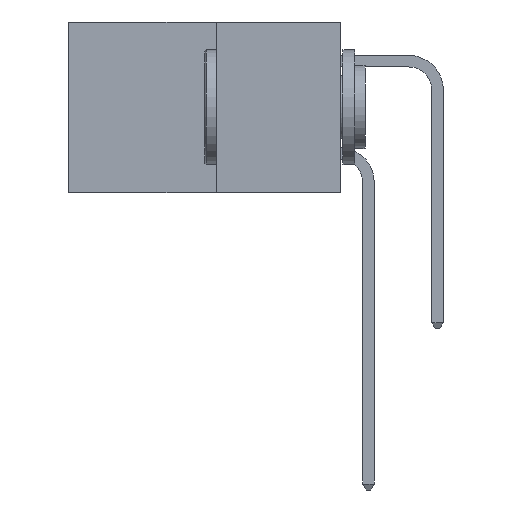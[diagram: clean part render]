
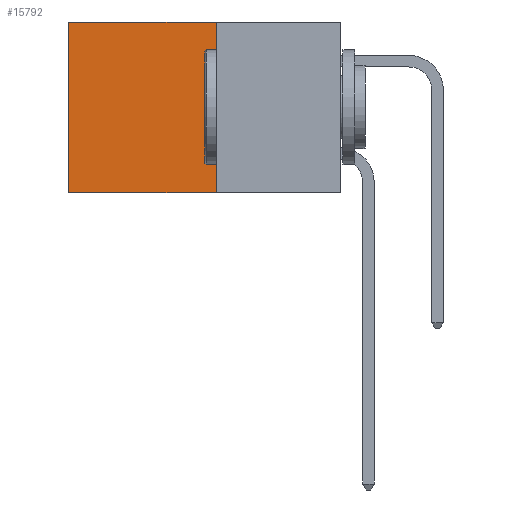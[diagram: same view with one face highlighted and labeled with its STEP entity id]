
A CAD part, left-side view. The second image highlights one B-rep face of the part: STEP entity #15792.
In plain terms, the highlighted planar face has unit normal (-1, 0, 0).
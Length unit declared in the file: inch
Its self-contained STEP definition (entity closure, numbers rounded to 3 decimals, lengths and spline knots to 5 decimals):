
#416 = LINE ( 'NONE', #24177, #5683 ) ;
#655 = EDGE_LOOP ( 'NONE', ( #22769, #10283, #16898, #8484 ) ) ;
#665 = EDGE_CURVE ( 'NONE', #13209, #21080, #22031, .T. ) ;
#1738 = VECTOR ( 'NONE', #3641, 39.37008 ) ;
#2071 = CARTESIAN_POINT ( 'NONE',  ( 0.277, 0.27, -0.37 ) ) ;
#2329 = AXIS2_PLACEMENT_3D ( 'NONE', #20616, #8903, #22527 ) ;
#2977 = PLANE ( 'NONE',  #2329 ) ;
#2993 = LINE ( 'NONE', #21242, #1738 ) ;
#3641 = DIRECTION ( 'NONE',  ( 0., 0., -1. ) ) ;
#4662 = CARTESIAN_POINT ( 'NONE',  ( 0.277, 0.59, -0.37 ) ) ;
#5683 = VECTOR ( 'NONE', #18418, 39.37008 ) ;
#6483 = EDGE_CURVE ( 'NONE', #21080, #21301, #16597, .T. ) ;
#8458 = DIRECTION ( 'NONE',  ( 0., 1., 0. ) ) ;
#8484 = ORIENTED_EDGE ( 'NONE', *, *, #20109, .T. ) ;
#8903 = DIRECTION ( 'NONE',  ( 1., 0., 0. ) ) ;
#10283 = ORIENTED_EDGE ( 'NONE', *, *, #6483, .F. ) ;
#10859 = DIRECTION ( 'NONE',  ( 0., 0., -1. ) ) ;
#12532 = CARTESIAN_POINT ( 'NONE',  ( 0.277, 0.27, 0. ) ) ;
#13209 = VERTEX_POINT ( 'NONE', #12532 ) ;
#13242 = CARTESIAN_POINT ( 'NONE',  ( 0.277, 0.27, -0.37 ) ) ;
#15792 = ADVANCED_FACE ( 'NONE', ( #24137 ), #2977, .F. ) ;
#16237 = VERTEX_POINT ( 'NONE', #17884 ) ;
#16597 = LINE ( 'NONE', #20183, #21749 ) ;
#16898 = ORIENTED_EDGE ( 'NONE', *, *, #665, .F. ) ;
#17884 = CARTESIAN_POINT ( 'NONE',  ( 0.277, 0.59, 0. ) ) ;
#18418 = DIRECTION ( 'NONE',  ( 0., 1., 0. ) ) ;
#18714 = EDGE_CURVE ( 'NONE', #16237, #21301, #2993, .T. ) ;
#20109 = EDGE_CURVE ( 'NONE', #13209, #16237, #416, .T. ) ;
#20183 = CARTESIAN_POINT ( 'NONE',  ( 0.277, 0.27, -0.37 ) ) ;
#20616 = CARTESIAN_POINT ( 'NONE',  ( 0.277, 0.27, -0.37 ) ) ;
#21080 = VERTEX_POINT ( 'NONE', #2071 ) ;
#21242 = CARTESIAN_POINT ( 'NONE',  ( 0.277, 0.59, -0.37 ) ) ;
#21301 = VERTEX_POINT ( 'NONE', #4662 ) ;
#21444 = VECTOR ( 'NONE', #10859, 39.37008 ) ;
#21749 = VECTOR ( 'NONE', #8458, 39.37008 ) ;
#22031 = LINE ( 'NONE', #13242, #21444 ) ;
#22527 = DIRECTION ( 'NONE',  ( 0., 0., -1. ) ) ;
#22769 = ORIENTED_EDGE ( 'NONE', *, *, #18714, .T. ) ;
#24137 = FACE_OUTER_BOUND ( 'NONE', #655, .T. ) ;
#24177 = CARTESIAN_POINT ( 'NONE',  ( 0.277, 0.27, 0. ) ) ;
